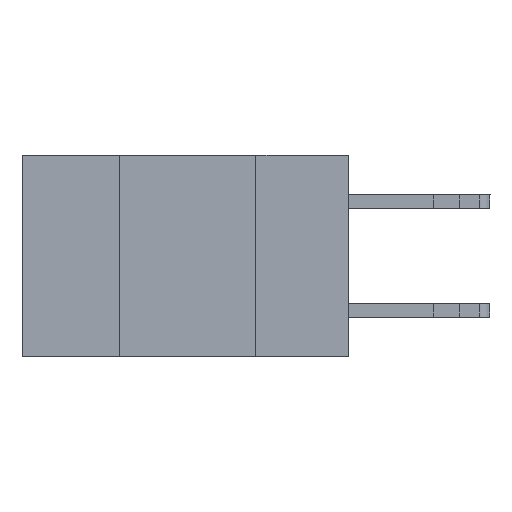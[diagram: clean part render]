
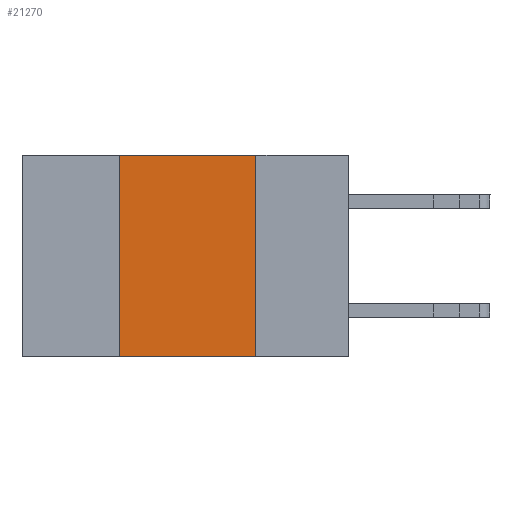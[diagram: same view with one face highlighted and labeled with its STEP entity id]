
A CAD part, left-side view. The second image highlights one B-rep face of the part: STEP entity #21270.
In plain terms, the highlighted planar face has unit normal (-1, 0, 0).
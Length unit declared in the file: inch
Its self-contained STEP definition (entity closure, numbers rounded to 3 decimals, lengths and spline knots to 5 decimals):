
#416 = LINE ( 'NONE', #7276, #5067 ) ;
#1761 = VERTEX_POINT ( 'NONE', #15363 ) ;
#2322 = VERTEX_POINT ( 'NONE', #16115 ) ;
#2599 = EDGE_CURVE ( 'NONE', #2322, #13239, #21009, .T. ) ;
#3031 = DIRECTION ( 'NONE',  ( 0., 0., -1. ) ) ;
#3395 = CARTESIAN_POINT ( 'NONE',  ( 0., 0.6, -0.37 ) ) ;
#3932 = CARTESIAN_POINT ( 'NONE',  ( 0., 0.42, 0. ) ) ;
#4843 = CARTESIAN_POINT ( 'NONE',  ( 0., 0.6, 0. ) ) ;
#5045 = VERTEX_POINT ( 'NONE', #15050 ) ;
#5067 = VECTOR ( 'NONE', #5594, 39.37008 ) ;
#5594 = DIRECTION ( 'NONE',  ( 0., 0., -1. ) ) ;
#6067 = DIRECTION ( 'NONE',  ( 1., 0., 0. ) ) ;
#6616 = VECTOR ( 'NONE', #12353, 39.37008 ) ;
#6849 = VECTOR ( 'NONE', #11918, 39.37008 ) ;
#7276 = CARTESIAN_POINT ( 'NONE',  ( 0., 0.17, 0. ) ) ;
#7521 = EDGE_CURVE ( 'NONE', #2322, #1761, #15299, .T. ) ;
#7654 = CARTESIAN_POINT ( 'NONE',  ( 0., 0.6, 0. ) ) ;
#8152 = CARTESIAN_POINT ( 'NONE',  ( 0., 0.42, 0. ) ) ;
#9111 = AXIS2_PLACEMENT_3D ( 'NONE', #7654, #6067, #3031 ) ;
#9771 = ORIENTED_EDGE ( 'NONE', *, *, #2599, .F. ) ;
#9799 = LINE ( 'NONE', #4843, #6849 ) ;
#10469 = ORIENTED_EDGE ( 'NONE', *, *, #18461, .F. ) ;
#11252 = FACE_OUTER_BOUND ( 'NONE', #18746, .T. ) ;
#11831 = ORIENTED_EDGE ( 'NONE', *, *, #7521, .T. ) ;
#11918 = DIRECTION ( 'NONE',  ( 0., -1., 0. ) ) ;
#12172 = ORIENTED_EDGE ( 'NONE', *, *, #16532, .F. ) ;
#12353 = DIRECTION ( 'NONE',  ( 0., 0., 1. ) ) ;
#13239 = VERTEX_POINT ( 'NONE', #8152 ) ;
#15050 = CARTESIAN_POINT ( 'NONE',  ( 0., 0.17, 0. ) ) ;
#15255 = PLANE ( 'NONE',  #9111 ) ;
#15299 = LINE ( 'NONE', #3395, #16431 ) ;
#15363 = CARTESIAN_POINT ( 'NONE',  ( 0., 0.17, -0.37 ) ) ;
#16115 = CARTESIAN_POINT ( 'NONE',  ( 0., 0.42, -0.37 ) ) ;
#16431 = VECTOR ( 'NONE', #16668, 39.37008 ) ;
#16532 = EDGE_CURVE ( 'NONE', #13239, #5045, #9799, .T. ) ;
#16668 = DIRECTION ( 'NONE',  ( 0., -1., 0. ) ) ;
#18461 = EDGE_CURVE ( 'NONE', #5045, #1761, #416, .T. ) ;
#18746 = EDGE_LOOP ( 'NONE', ( #10469, #12172, #9771, #11831 ) ) ;
#21009 = LINE ( 'NONE', #3932, #6616 ) ;
#21270 = ADVANCED_FACE ( 'NONE', ( #11252 ), #15255, .F. ) ;
